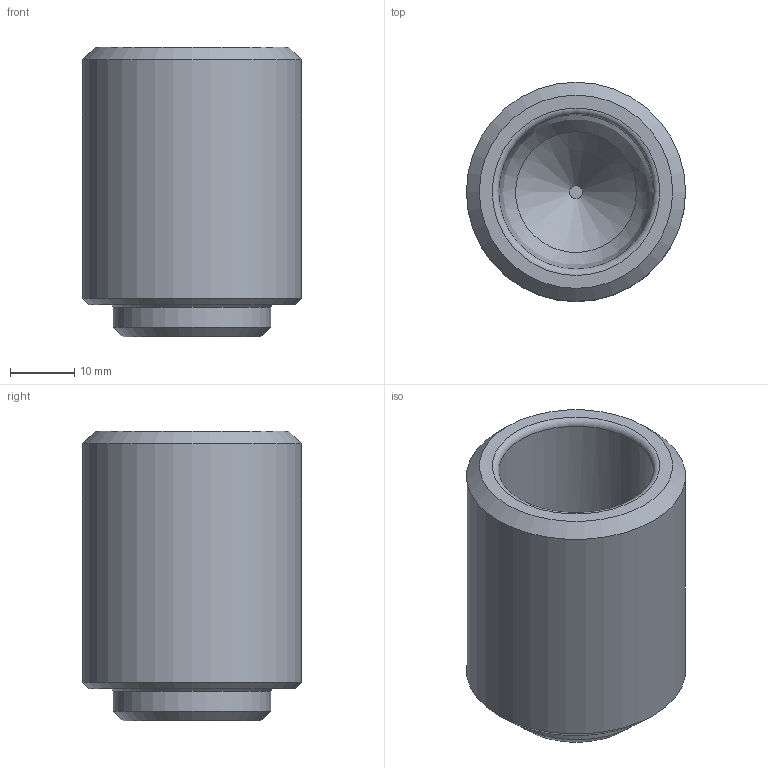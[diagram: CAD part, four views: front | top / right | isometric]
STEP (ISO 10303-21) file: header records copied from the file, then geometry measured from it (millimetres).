
FILE_DESCRIPTION(('FreeCAD Model'),'2;1');
FILE_NAME('Open CASCADE Shape Model','2022-10-05T16:34:58',('Author'),( ''),'Open CASCADE STEP processor 7.6','FreeCAD','Unknown');
FILE_SCHEMA(('AUTOMOTIVE_DESIGN { 1 0 10303 214 1 1 1 1 }'));
Length unit declared in the file: millimetre
Products named in the file (1): Projectile - Long
Bounding box: 34 x 34 x 45 mm (x, y, z)
Volume: 25151.2 mm3; surface area: 8221.4 mm2
Topology: 1 solids, 1 shells, 14 faces, 23 edges, 13 vertices
Faces by surface type: cone 5, plane 4, cylinder 3, torus 1, bspline 1
Full cylindrical faces by diameter (mm): 24 x1, 24.4 x1, 34 x1
Entity records: 747 total; most frequent: CARTESIAN_POINT 245, DIRECTION 90, ORIENTED_EDGE 46, PCURVE 46, DEFINITIONAL_REPRESENTATION 46, LINE 32, VECTOR 32, AXIS2_PLACEMENT_3D 26
